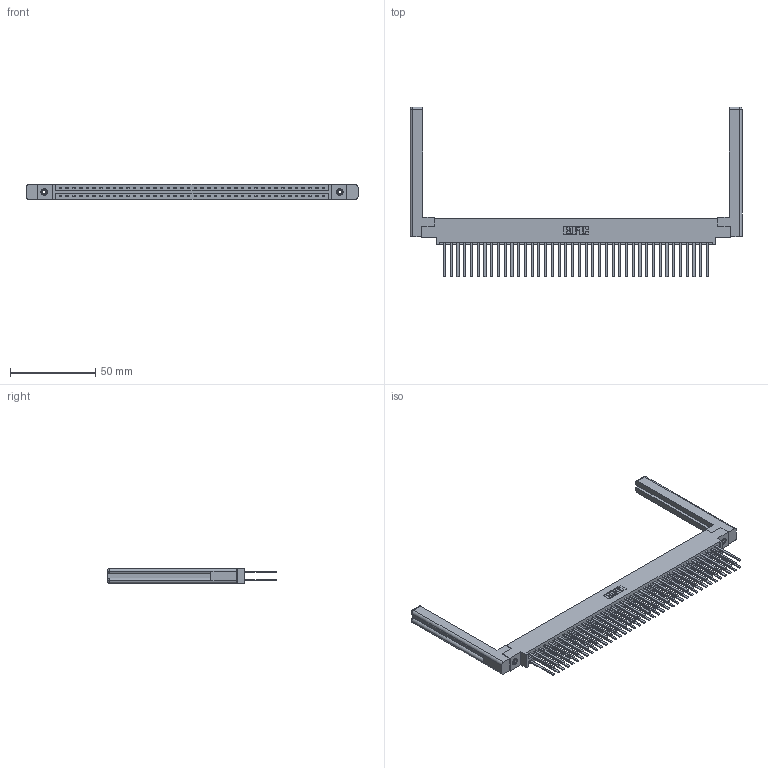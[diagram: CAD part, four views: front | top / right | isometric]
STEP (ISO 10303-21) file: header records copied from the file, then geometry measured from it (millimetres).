
FILE_DESCRIPTION (( 'STEP AP203' ), '1' );
FILE_NAME ('387-080-544-858.STEP', '2019-10-22T22:29:18', ( '' ), ( '' ), 'SwSTEP 2.0', 'SolidWorks 2016', '' );
FILE_SCHEMA (( 'CONFIG_CONTROL_DESIGN' ));
Length unit declared in the file: inch
Products named in the file (5): 387-080-544-858; 345-250-001_345-250-001-102; 337 Part_0.170 Offset - 0.156 Dia-TI; 307-220-058; 345-292-001_345-293-144
Assembly tree (85 placements, depth 2):
  387-080-544-858
    337 Part_0.170 Offset - 0.156 Dia-TI
    345-292-001_345-293-144  x80
    345-250-001_345-250-001-102  x2
    307-220-058  x2
Bounding box: 195.12 x 99.7 x 9.4 mm (x, y, z)
Volume: 28683.3 mm3; surface area: 33150.7 mm2
Topology: 85 solids, 85 shells, 4100 faces, 12117 edges, 7958 vertices
Faces by surface type: plane 2878, cylinder 1198, cone 12, torus 12
Entity records: 33854 total; most frequent: CARTESIAN_POINT 5713, ORIENTED_EDGE 5588, DIRECTION 4874, EDGE_CURVE 2794, VECTOR 2622, LINE 2622, VERTEX_POINT 1854, AXIS2_PLACEMENT_3D 1126
